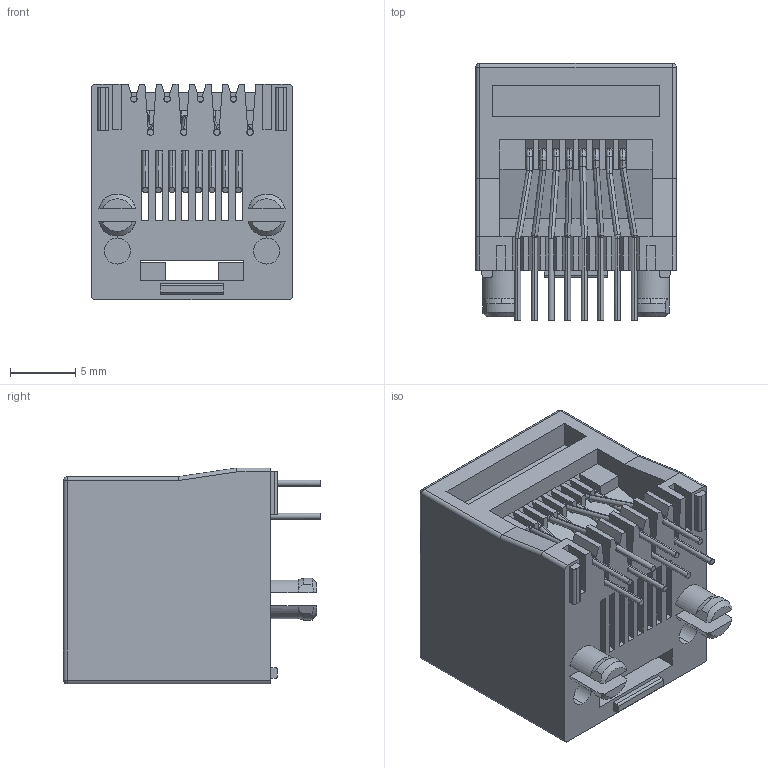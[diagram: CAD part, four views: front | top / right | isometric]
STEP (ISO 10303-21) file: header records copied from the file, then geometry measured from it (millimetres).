
FILE_DESCRIPTION (( 'STEP AP203' ), '1' );
FILE_NAME ('RJ20018831P00031.STEP', '2020-01-15T15:59:57', ( '' ), ( '' ), 'SwSTEP 2.0', 'SolidWorks 2016', '' );
FILE_SCHEMA (( 'CONFIG_CONTROL_DESIGN' ));
Length unit declared in the file: millimetre
Products named in the file (3): RJ20018831P00031; 20 Contacts; 20 Insulator
Assembly tree (2 placements, depth 2):
  RJ20018831P00031
    20 Insulator
    20 Contacts
Bounding box: 15.36 x 19.68 x 16.54 mm (x, y, z)
Volume: 1934.9 mm3; surface area: 3110.1 mm2
Topology: 9 solids, 9 shells, 573 faces, 1536 edges, 967 vertices
Faces by surface type: plane 332, cylinder 193, bspline 36, cone 12
Entity records: 19874 total; most frequent: CARTESIAN_POINT 5625, ORIENTED_EDGE 3072, DIRECTION 2737, EDGE_CURVE 1536, VECTOR 1057, LINE 1057, VERTEX_POINT 967, AXIS2_PLACEMENT_3D 840
